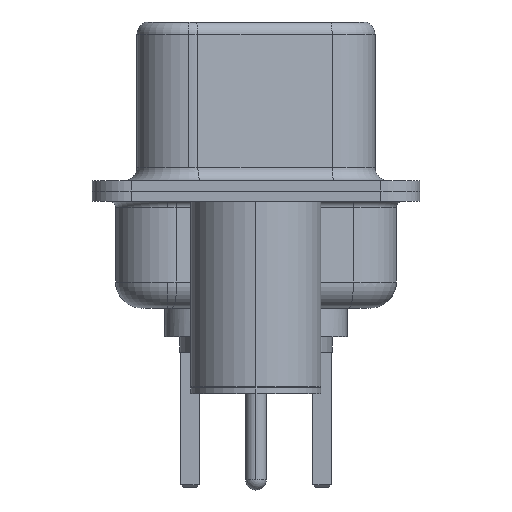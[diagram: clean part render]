
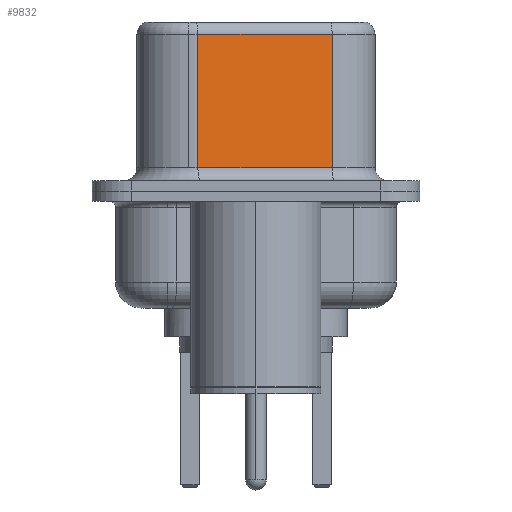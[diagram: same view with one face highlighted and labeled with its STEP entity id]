
A CAD part, left-side view. The second image highlights one B-rep face of the part: STEP entity #9832.
In plain terms, the highlighted planar face has unit normal (-0.985, -0.174, 0).
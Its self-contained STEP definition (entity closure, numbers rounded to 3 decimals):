
#932 = ORIENTED_EDGE ( 'NONE', *, *, #6848, .T. ) ;
#939 = DIRECTION ( 'NONE',  ( 0.174, -0.985, 0. ) ) ;
#2774 = VECTOR ( 'NONE', #5149, 1000. ) ;
#2997 = EDGE_CURVE ( 'NONE', #3649, #12139, #13929, .T. ) ;
#3148 = EDGE_LOOP ( 'NONE', ( #13153, #932, #18479, #5834 ) ) ;
#3649 = VERTEX_POINT ( 'NONE', #17167 ) ;
#3697 = DIRECTION ( 'NONE',  ( 0.985, 0.174, 0. ) ) ;
#5149 = DIRECTION ( 'NONE',  ( 0., 0., -1. ) ) ;
#5834 = ORIENTED_EDGE ( 'NONE', *, *, #14184, .T. ) ;
#6617 = VECTOR ( 'NONE', #14127, 1000. ) ;
#6753 = CARTESIAN_POINT ( 'NONE',  ( 4.58, -2.927, 0.9 ) ) ;
#6848 = EDGE_CURVE ( 'NONE', #12792, #3649, #11829, .T. ) ;
#7471 = VECTOR ( 'NONE', #9277, 1000. ) ;
#7498 = FACE_OUTER_BOUND ( 'NONE', #3148, .T. ) ;
#8064 = LINE ( 'NONE', #6753, #11483 ) ;
#9277 = DIRECTION ( 'NONE',  ( -0.174, 0.985, 0. ) ) ;
#9350 = VERTEX_POINT ( 'NONE', #16972 ) ;
#9406 = CARTESIAN_POINT ( 'NONE',  ( 4.58, -2.927, 6.52 ) ) ;
#9811 = CARTESIAN_POINT ( 'NONE',  ( 4.58, -2.927, 6.52 ) ) ;
#9832 = ADVANCED_FACE ( 'NONE', ( #7498 ), #16640, .F. ) ;
#11483 = VECTOR ( 'NONE', #939, 1000. ) ;
#11775 = EDGE_CURVE ( 'NONE', #12792, #9350, #16727, .T. ) ;
#11829 = LINE ( 'NONE', #16582, #7471 ) ;
#12139 = VERTEX_POINT ( 'NONE', #14716 ) ;
#12792 = VERTEX_POINT ( 'NONE', #13405 ) ;
#13153 = ORIENTED_EDGE ( 'NONE', *, *, #11775, .F. ) ;
#13405 = CARTESIAN_POINT ( 'NONE',  ( 4.58, -2.927, 6.02 ) ) ;
#13809 = DIRECTION ( 'NONE',  ( -0.174, 0.985, 0. ) ) ;
#13929 = LINE ( 'NONE', #15919, #2774 ) ;
#14127 = DIRECTION ( 'NONE',  ( 0., 0., -1. ) ) ;
#14184 = EDGE_CURVE ( 'NONE', #12139, #9350, #8064, .T. ) ;
#14716 = CARTESIAN_POINT ( 'NONE',  ( 3.67, 2.233, 0.9 ) ) ;
#15919 = CARTESIAN_POINT ( 'NONE',  ( 3.67, 2.233, 6.52 ) ) ;
#16582 = CARTESIAN_POINT ( 'NONE',  ( 4.58, -2.927, 6.02 ) ) ;
#16640 = PLANE ( 'NONE',  #18387 ) ;
#16727 = LINE ( 'NONE', #9811, #6617 ) ;
#16972 = CARTESIAN_POINT ( 'NONE',  ( 4.58, -2.927, 0.9 ) ) ;
#17167 = CARTESIAN_POINT ( 'NONE',  ( 3.67, 2.233, 6.02 ) ) ;
#18387 = AXIS2_PLACEMENT_3D ( 'NONE', #9406, #3697, #13809 ) ;
#18479 = ORIENTED_EDGE ( 'NONE', *, *, #2997, .T. ) ;
